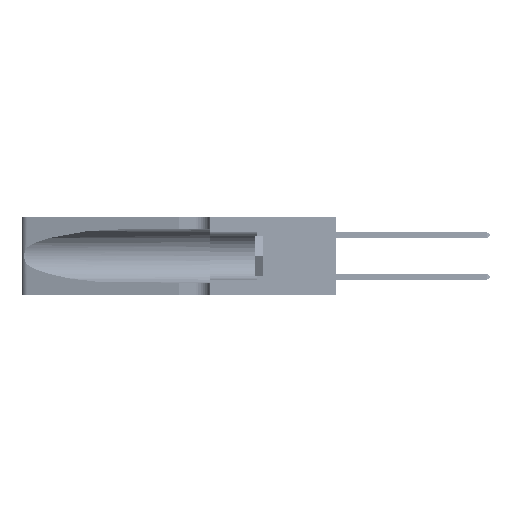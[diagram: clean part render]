
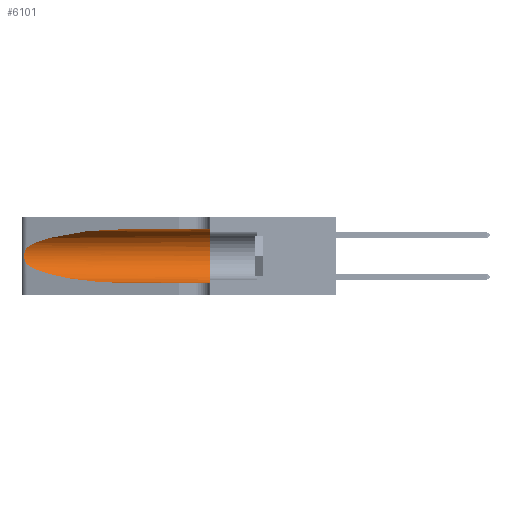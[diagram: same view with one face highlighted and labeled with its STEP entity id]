
A CAD part, left-side view. The second image highlights one B-rep face of the part: STEP entity #6101.
In plain terms, the highlighted cylindrical face has radius 3.308 mm (diameter 6.617 mm), a partial arc.
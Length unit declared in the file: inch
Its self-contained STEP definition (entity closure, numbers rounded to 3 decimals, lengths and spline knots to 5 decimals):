
#1101 = ORIENTED_EDGE ( 'NONE', *, *, #22890, .T. ) ;
#1114 = FACE_OUTER_BOUND ( 'NONE', #20453, .T. ) ;
#1271 = CARTESIAN_POINT ( 'NONE',  ( 0.1305, 1.61858, 0.05475 ) ) ;
#2142 = CARTESIAN_POINT ( 'NONE',  ( 0.25487, 1.22718, 0.22369 ) ) ;
#3037 = CARTESIAN_POINT ( 'NONE',  ( 0.1305, 0.72297, 0.05475 ) ) ;
#3380 = CARTESIAN_POINT ( 'NONE',  ( 0.26075, 1.23896, 0.178 ) ) ;
#3816 = CARTESIAN_POINT ( 'NONE',  ( 0.1305, 0.35, 0.185 ) ) ;
#5142 = AXIS2_PLACEMENT_3D ( 'NONE', #3816, #32736, #7955 ) ;
#5453 = CIRCLE ( 'NONE', #5142, 0.13025 ) ;
#6101 = ADVANCED_FACE ( 'NONE', ( #1114 ), #42398, .F. ) ;
#6442 = B_SPLINE_CURVE_WITH_KNOTS ( 'NONE', 3,
 ( #44530, #15728, #40397, #48665, #24063, #52775, #28227, #3380, #32341, #7543, #36443, #11713, #40580, #15908 ),
 .UNSPECIFIED., .F., .F.,
 ( 4, 2, 2, 2, 2, 2, 4 ),
 ( 0., 0.00027, 0.00053, 0.00107, 0.0016, 0.00187, 0.00214 ),
 .UNSPECIFIED. ) ;
#7058 = EDGE_CURVE ( 'NONE', #33133, #35886, #9925, .T. ) ;
#7391 = EDGE_CURVE ( 'NONE', #35129, #9552, #6442, .T. ) ;
#7470 = CARTESIAN_POINT ( 'NONE',  ( 0.1305, 0.72297, 0.05475 ) ) ;
#7543 = CARTESIAN_POINT ( 'NONE',  ( 0.25856, 1.23593, 0.16098 ) ) ;
#7955 = DIRECTION ( 'NONE',  ( 0., 0., 1. ) ) ;
#7994 = ORIENTED_EDGE ( 'NONE', *, *, #7058, .T. ) ;
#9284 = LINE ( 'NONE', #34489, #31349 ) ;
#9552 = VERTEX_POINT ( 'NONE', #29623 ) ;
#9925 = LINE ( 'NONE', #1271, #41587 ) ;
#10076 = CARTESIAN_POINT ( 'NONE',  ( 0.1305, 0.35, 0.31525 ) ) ;
#11713 = CARTESIAN_POINT ( 'NONE',  ( 0.25639, 1.23186, 0.15144 ) ) ;
#13744 = DIRECTION ( 'NONE',  ( 0., -1., 0. ) ) ;
#15728 = CARTESIAN_POINT ( 'NONE',  ( 0.25555, 1.22994, 0.2215 ) ) ;
#15908 = CARTESIAN_POINT ( 'NONE',  ( 0.25487, 1.22718, 0.14631 ) ) ;
#16644 = CARTESIAN_POINT ( 'NONE',  ( 0.25487, 1.22718, 0.22369 ) ) ;
#20453 = EDGE_LOOP ( 'NONE', ( #27532, #23640, #1101, #7994, #33626, #36922 ) ) ;
#21456 = CARTESIAN_POINT ( 'NONE',  ( 0.1305, 0.35, 0.05475 ) ) ;
#22890 = EDGE_CURVE ( 'NONE', #9552, #33133, #40518, .T. ) ;
#23556 = CARTESIAN_POINT ( 'NONE',  ( 0.2373, 1.15595, 0.08982 ) ) ;
#23640 = ORIENTED_EDGE ( 'NONE', *, *, #7391, .T. ) ;
#23733 = CARTESIAN_POINT ( 'NONE',  ( 0.25487, 1.22718, 0.14631 ) ) ;
#24063 = CARTESIAN_POINT ( 'NONE',  ( 0.25854, 1.2359, 0.20912 ) ) ;
#24741 = CARTESIAN_POINT ( 'NONE',  ( 0.1305, 0.72297, 0.31525 ) ) ;
#24953 = AXIS2_PLACEMENT_3D ( 'NONE', #24996, #33082, #29153 ) ;
#24996 = CARTESIAN_POINT ( 'NONE',  ( 0.1305, 1.61858, 0.185 ) ) ;
#25324 = EDGE_CURVE ( 'NONE', #37988, #35129, #37546, .T. ) ;
#26778 = CARTESIAN_POINT ( 'NONE',  ( 0.1305, 0.72297, 0.31525 ) ) ;
#26963 = CARTESIAN_POINT ( 'NONE',  ( 0.2373, 1.15595, 0.28018 ) ) ;
#27532 = ORIENTED_EDGE ( 'NONE', *, *, #25324, .T. ) ;
#27899 = CARTESIAN_POINT ( 'NONE',  ( 0.18966, 0.96281, 0.05475 ) ) ;
#28227 = CARTESIAN_POINT ( 'NONE',  ( 0.26075, 1.23896, 0.19203 ) ) ;
#29153 = DIRECTION ( 'NONE',  ( 0., 0., -1. ) ) ;
#29623 = CARTESIAN_POINT ( 'NONE',  ( 0.25487, 1.22718, 0.14631 ) ) ;
#30235 = EDGE_CURVE ( 'NONE', #37988, #34122, #9284, .T. ) ;
#31349 = VECTOR ( 'NONE', #38618, 39.37008 ) ;
#32341 = CARTESIAN_POINT ( 'NONE',  ( 0.26017, 1.23833, 0.17102 ) ) ;
#32736 = DIRECTION ( 'NONE',  ( 0., 1., 0. ) ) ;
#33082 = DIRECTION ( 'NONE',  ( 0., -1., 0. ) ) ;
#33133 = VERTEX_POINT ( 'NONE', #7470 ) ;
#33626 = ORIENTED_EDGE ( 'NONE', *, *, #43843, .F. ) ;
#34122 = VERTEX_POINT ( 'NONE', #10076 ) ;
#34489 = CARTESIAN_POINT ( 'NONE',  ( 0.1305, 1.61858, 0.31525 ) ) ;
#35129 = VERTEX_POINT ( 'NONE', #16644 ) ;
#35886 = VERTEX_POINT ( 'NONE', #21456 ) ;
#36443 = CARTESIAN_POINT ( 'NONE',  ( 0.25789, 1.23486, 0.15765 ) ) ;
#36922 = ORIENTED_EDGE ( 'NONE', *, *, #30235, .F. ) ;
#37546 =( BOUNDED_CURVE ( )  B_SPLINE_CURVE ( 3, ( #26778, #47400, #26963, #2142 ),
 .UNSPECIFIED., .F., .T. ) 
 B_SPLINE_CURVE_WITH_KNOTS ( ( 4, 4 ),
 ( 1.5708, 2.84003 ),
 .UNSPECIFIED. ) 
 CURVE ( )  GEOMETRIC_REPRESENTATION_ITEM ( )  RATIONAL_B_SPLINE_CURVE ( ( 1., 0.87, 0.87, 1. ) ) 
 REPRESENTATION_ITEM ( '' )  );
#37988 = VERTEX_POINT ( 'NONE', #24741 ) ;
#38618 = DIRECTION ( 'NONE',  ( 0., -1., 0. ) ) ;
#40397 = CARTESIAN_POINT ( 'NONE',  ( 0.25639, 1.23184, 0.21858 ) ) ;
#40518 =( BOUNDED_CURVE ( )  B_SPLINE_CURVE ( 3, ( #23733, #23556, #27899, #3037 ),
 .UNSPECIFIED., .F., .F. ) 
 B_SPLINE_CURVE_WITH_KNOTS ( ( 4, 4 ),
 ( 3.44316, 4.71239 ),
 .UNSPECIFIED. ) 
 CURVE ( )  GEOMETRIC_REPRESENTATION_ITEM ( )  RATIONAL_B_SPLINE_CURVE ( ( 1., 0.87, 0.87, 1. ) ) 
 REPRESENTATION_ITEM ( '' )  );
#40580 = CARTESIAN_POINT ( 'NONE',  ( 0.25555, 1.22993, 0.14849 ) ) ;
#41587 = VECTOR ( 'NONE', #13744, 39.37008 ) ;
#42398 = CYLINDRICAL_SURFACE ( 'NONE', #24953, 0.13025 ) ;
#43843 = EDGE_CURVE ( 'NONE', #34122, #35886, #5453, .T. ) ;
#44530 = CARTESIAN_POINT ( 'NONE',  ( 0.25487, 1.22718, 0.22369 ) ) ;
#47400 = CARTESIAN_POINT ( 'NONE',  ( 0.18966, 0.96281, 0.31525 ) ) ;
#48665 = CARTESIAN_POINT ( 'NONE',  ( 0.25787, 1.23484, 0.2124 ) ) ;
#52775 = CARTESIAN_POINT ( 'NONE',  ( 0.26018, 1.23835, 0.19895 ) ) ;
